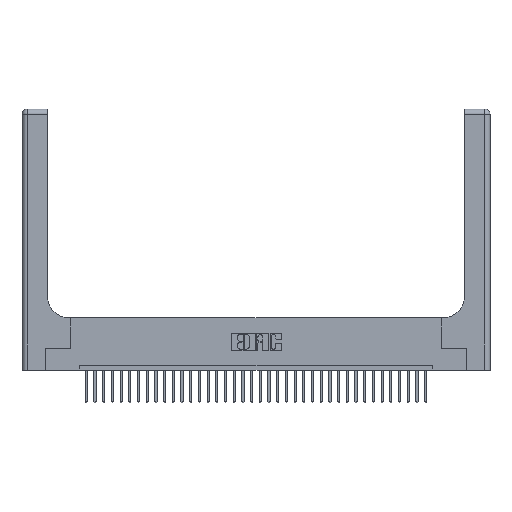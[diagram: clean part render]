
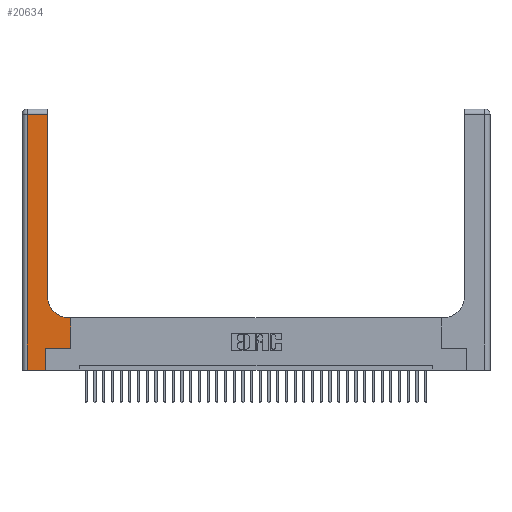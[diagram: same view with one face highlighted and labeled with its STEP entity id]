
A CAD part, top view. The second image highlights one B-rep face of the part: STEP entity #20634.
In plain terms, the highlighted planar face has unit normal (0, 0, 1).
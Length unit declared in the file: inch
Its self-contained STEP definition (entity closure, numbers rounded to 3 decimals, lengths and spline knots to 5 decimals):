
#227 = CARTESIAN_POINT ( 'NONE',  ( 0.06, 0., 0.37 ) ) ;
#329 = LINE ( 'NONE', #7025, #5941 ) ;
#374 = VERTEX_POINT ( 'NONE', #32295 ) ;
#888 = ORIENTED_EDGE ( 'NONE', *, *, #30194, .T. ) ;
#1083 = LINE ( 'NONE', #25714, #14475 ) ;
#1666 = EDGE_CURVE ( 'NONE', #27916, #13193, #19712, .T. ) ;
#1996 = VERTEX_POINT ( 'NONE', #34934 ) ;
#2132 = ORIENTED_EDGE ( 'NONE', *, *, #20138, .T. ) ;
#2162 = LINE ( 'NONE', #21033, #9021 ) ;
#2172 = EDGE_CURVE ( 'NONE', #374, #17571, #34241, .T. ) ;
#2278 = ORIENTED_EDGE ( 'NONE', *, *, #30372, .T. ) ;
#4272 = CARTESIAN_POINT ( 'NONE',  ( 0., 2.94, 0.37 ) ) ;
#4377 = DIRECTION ( 'NONE',  ( 0., -1., 0. ) ) ;
#5340 = CARTESIAN_POINT ( 'NONE',  ( 0.5415, 0.6, 0.37 ) ) ;
#5468 = AXIS2_PLACEMENT_3D ( 'NONE', #17188, #5935, #33304 ) ;
#5935 = DIRECTION ( 'NONE',  ( 0., 0., -1. ) ) ;
#5941 = VECTOR ( 'NONE', #4377, 39.37008 ) ;
#6841 = VERTEX_POINT ( 'NONE', #27968 ) ;
#7025 = CARTESIAN_POINT ( 'NONE',  ( 0.06, 3., 0.37 ) ) ;
#7607 = DIRECTION ( 'NONE',  ( 0., 1., 0. ) ) ;
#8424 = AXIS2_PLACEMENT_3D ( 'NONE', #23111, #13321, #26719 ) ;
#9021 = VECTOR ( 'NONE', #26153, 39.37008 ) ;
#9113 = CARTESIAN_POINT ( 'NONE',  ( 0.2915, 2.94, 0.37 ) ) ;
#9185 = VECTOR ( 'NONE', #33099, 39.37008 ) ;
#9282 = EDGE_CURVE ( 'NONE', #27128, #1996, #22764, .T. ) ;
#10385 = ORIENTED_EDGE ( 'NONE', *, *, #21747, .T. ) ;
#10635 = EDGE_CURVE ( 'NONE', #13193, #14041, #18763, .T. ) ;
#11022 = CARTESIAN_POINT ( 'NONE',  ( 0.2915, 0.85, 0.37 ) ) ;
#12626 = CARTESIAN_POINT ( 'NONE',  ( 0.2915, 0.6, 0.37 ) ) ;
#13054 = CARTESIAN_POINT ( 'NONE',  ( 0.2915, 3., 0.37 ) ) ;
#13126 = DIRECTION ( 'NONE',  ( 1., 0., 0. ) ) ;
#13193 = VERTEX_POINT ( 'NONE', #9113 ) ;
#13321 = DIRECTION ( 'NONE',  ( 0., 0., -1. ) ) ;
#14039 = VECTOR ( 'NONE', #26641, 39.37008 ) ;
#14041 = VERTEX_POINT ( 'NONE', #31277 ) ;
#14475 = VECTOR ( 'NONE', #28234, 39.37008 ) ;
#16585 = VERTEX_POINT ( 'NONE', #25063 ) ;
#17188 = CARTESIAN_POINT ( 'NONE',  ( 0., 3., 0.37 ) ) ;
#17571 = VERTEX_POINT ( 'NONE', #5340 ) ;
#17783 = CIRCLE ( 'NONE', #8424, 0.25 ) ;
#17852 = ORIENTED_EDGE ( 'NONE', *, *, #1666, .T. ) ;
#18763 = LINE ( 'NONE', #4272, #14039 ) ;
#19321 = ORIENTED_EDGE ( 'NONE', *, *, #28694, .T. ) ;
#19712 = LINE ( 'NONE', #13054, #35571 ) ;
#20138 = EDGE_CURVE ( 'NONE', #14041, #27128, #329, .T. ) ;
#20288 = ORIENTED_EDGE ( 'NONE', *, *, #9282, .T. ) ;
#20634 = ADVANCED_FACE ( 'NONE', ( #21416 ), #22408, .F. ) ;
#21033 = CARTESIAN_POINT ( 'NONE',  ( 0.269, 0., 0.37 ) ) ;
#21416 = FACE_OUTER_BOUND ( 'NONE', #32888, .T. ) ;
#21747 = EDGE_CURVE ( 'NONE', #16585, #374, #1083, .T. ) ;
#22408 = PLANE ( 'NONE',  #5468 ) ;
#22764 = LINE ( 'NONE', #26993, #27475 ) ;
#23111 = CARTESIAN_POINT ( 'NONE',  ( 0.5415, 0.85, 0.37 ) ) ;
#23535 = DIRECTION ( 'NONE',  ( -1., 0., 0. ) ) ;
#24654 = LINE ( 'NONE', #32988, #9185 ) ;
#25063 = CARTESIAN_POINT ( 'NONE',  ( 0.5585, 0.25, 0.37 ) ) ;
#25714 = CARTESIAN_POINT ( 'NONE',  ( 0.5585, 0.25, 0.37 ) ) ;
#26153 = DIRECTION ( 'NONE',  ( 0., 1., 0. ) ) ;
#26641 = DIRECTION ( 'NONE',  ( -1., 0., 0. ) ) ;
#26719 = DIRECTION ( 'NONE',  ( 1., 0., 0. ) ) ;
#26993 = CARTESIAN_POINT ( 'NONE',  ( 0., 0., 0.37 ) ) ;
#27128 = VERTEX_POINT ( 'NONE', #227 ) ;
#27475 = VECTOR ( 'NONE', #13126, 39.37008 ) ;
#27916 = VERTEX_POINT ( 'NONE', #11022 ) ;
#27968 = CARTESIAN_POINT ( 'NONE',  ( 0.269, 0.25, 0.37 ) ) ;
#28234 = DIRECTION ( 'NONE',  ( 0., 1., 0. ) ) ;
#28694 = EDGE_CURVE ( 'NONE', #1996, #6841, #2162, .T. ) ;
#30194 = EDGE_CURVE ( 'NONE', #6841, #16585, #24654, .T. ) ;
#30372 = EDGE_CURVE ( 'NONE', #17571, #27916, #17783, .T. ) ;
#30778 = ORIENTED_EDGE ( 'NONE', *, *, #10635, .T. ) ;
#31277 = CARTESIAN_POINT ( 'NONE',  ( 0.06, 2.94, 0.37 ) ) ;
#32295 = CARTESIAN_POINT ( 'NONE',  ( 0.5585, 0.6, 0.37 ) ) ;
#32888 = EDGE_LOOP ( 'NONE', ( #17852, #30778, #2132, #20288, #19321, #888, #10385, #32936, #2278 ) ) ;
#32936 = ORIENTED_EDGE ( 'NONE', *, *, #2172, .T. ) ;
#32988 = CARTESIAN_POINT ( 'NONE',  ( 0.269, 0.25, 0.37 ) ) ;
#33099 = DIRECTION ( 'NONE',  ( 1., 0., 0. ) ) ;
#33304 = DIRECTION ( 'NONE',  ( -1., 0., 0. ) ) ;
#33820 = VECTOR ( 'NONE', #23535, 39.37008 ) ;
#34241 = LINE ( 'NONE', #12626, #33820 ) ;
#34934 = CARTESIAN_POINT ( 'NONE',  ( 0.269, 0., 0.37 ) ) ;
#35571 = VECTOR ( 'NONE', #7607, 39.37008 ) ;
